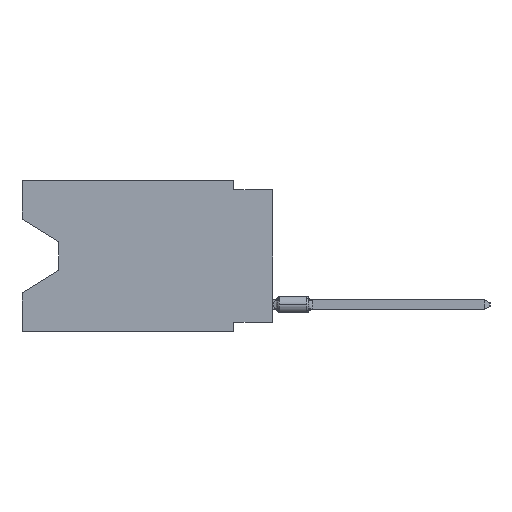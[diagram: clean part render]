
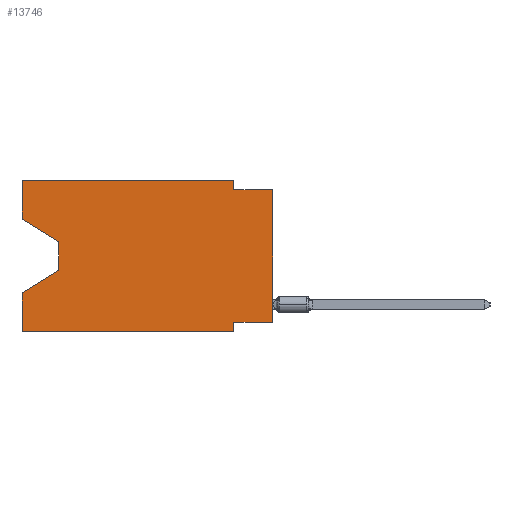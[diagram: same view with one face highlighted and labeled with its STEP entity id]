
A CAD part, left-side view. The second image highlights one B-rep face of the part: STEP entity #13746.
In plain terms, the highlighted planar face has unit normal (-1, 0, 0).
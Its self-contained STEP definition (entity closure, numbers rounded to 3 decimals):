
#204 = EDGE_CURVE ( 'NONE', #26065, #12717, #15722, .T. ) ;
#602 = VECTOR ( 'NONE', #33238, 1000. ) ;
#1590 = EDGE_CURVE ( 'NONE', #5926, #28278, #15044, .T. ) ;
#2101 = EDGE_CURVE ( 'NONE', #50760, #26065, #24980, .T. ) ;
#3023 = AXIS2_PLACEMENT_3D ( 'NONE', #23060, #48214, #26998 ) ;
#3065 = DIRECTION ( 'NONE',  ( 0., 1., 0. ) ) ;
#4132 = LINE ( 'NONE', #46897, #46453 ) ;
#4721 = ORIENTED_EDGE ( 'NONE', *, *, #204, .F. ) ;
#4770 = VECTOR ( 'NONE', #36698, 1000. ) ;
#5926 = VERTEX_POINT ( 'NONE', #23640 ) ;
#6097 = ORIENTED_EDGE ( 'NONE', *, *, #40734, .F. ) ;
#6844 = CARTESIAN_POINT ( 'NONE',  ( 0., 13.97, -5.893 ) ) ;
#7100 = ORIENTED_EDGE ( 'NONE', *, *, #37343, .T. ) ;
#8194 = DIRECTION ( 'NONE',  ( 0., -1., 0. ) ) ;
#9014 = DIRECTION ( 'NONE',  ( 0., 0., 1. ) ) ;
#9895 = EDGE_CURVE ( 'NONE', #27994, #50760, #37252, .T. ) ;
#10407 = CARTESIAN_POINT ( 'NONE',  ( 0., 0., -0.635 ) ) ;
#11821 = VECTOR ( 'NONE', #27916, 1000. ) ;
#12717 = VERTEX_POINT ( 'NONE', #54049 ) ;
#13085 = VERTEX_POINT ( 'NONE', #15163 ) ;
#13746 = ADVANCED_FACE ( 'NONE', ( #22240 ), #35372, .F. ) ;
#13950 = VECTOR ( 'NONE', #35538, 1000. ) ;
#14761 = CARTESIAN_POINT ( 'NONE',  ( 0., 0., -9.271 ) ) ;
#15003 = CARTESIAN_POINT ( 'NONE',  ( 0., 16.383, -9.906 ) ) ;
#15044 = LINE ( 'NONE', #49144, #11821 ) ;
#15163 = CARTESIAN_POINT ( 'NONE',  ( 0., 16.383, -2.546 ) ) ;
#15722 = LINE ( 'NONE', #10407, #52615 ) ;
#15752 = EDGE_CURVE ( 'NONE', #36811, #12717, #52286, .T. ) ;
#16286 = EDGE_CURVE ( 'NONE', #34697, #36162, #45864, .T. ) ;
#16830 = LINE ( 'NONE', #29154, #26396 ) ;
#16889 = VECTOR ( 'NONE', #38803, 1000. ) ;
#17072 = DIRECTION ( 'NONE',  ( 0., 0.855, -0.519 ) ) ;
#17743 = VECTOR ( 'NONE', #3065, 1000. ) ;
#20670 = DIRECTION ( 'NONE',  ( 0., 0., -1. ) ) ;
#21478 = LINE ( 'NONE', #42978, #16889 ) ;
#21681 = CARTESIAN_POINT ( 'NONE',  ( 0., 2.54, -9.906 ) ) ;
#21922 = ORIENTED_EDGE ( 'NONE', *, *, #9895, .F. ) ;
#22240 = FACE_OUTER_BOUND ( 'NONE', #24081, .T. ) ;
#22448 = VECTOR ( 'NONE', #28896, 1000. ) ;
#23060 = CARTESIAN_POINT ( 'NONE',  ( 0., 16.383, 0. ) ) ;
#23640 = CARTESIAN_POINT ( 'NONE',  ( 0., 2.54, -9.271 ) ) ;
#23828 = EDGE_CURVE ( 'NONE', #13085, #27994, #33508, .T. ) ;
#24081 = EDGE_LOOP ( 'NONE', ( #49636, #44207, #44071, #53375, #7100, #49864, #6097, #50116, #4721, #31886, #21922, #29466 ) ) ;
#24980 = LINE ( 'NONE', #37564, #22448 ) ;
#25000 = EDGE_CURVE ( 'NONE', #39496, #36162, #29987, .T. ) ;
#25499 = CARTESIAN_POINT ( 'NONE',  ( 0., 16.383, -7.36 ) ) ;
#26065 = VERTEX_POINT ( 'NONE', #30786 ) ;
#26396 = VECTOR ( 'NONE', #8194, 1000. ) ;
#26998 = DIRECTION ( 'NONE',  ( 0., 0., -1. ) ) ;
#27572 = CARTESIAN_POINT ( 'NONE',  ( 0., 16.383, 0. ) ) ;
#27916 = DIRECTION ( 'NONE',  ( 0., 0., -1. ) ) ;
#27994 = VERTEX_POINT ( 'NONE', #27572 ) ;
#28029 = CARTESIAN_POINT ( 'NONE',  ( 0., 16.383, 0. ) ) ;
#28278 = VERTEX_POINT ( 'NONE', #21681 ) ;
#28896 = DIRECTION ( 'NONE',  ( 0., 0., -1. ) ) ;
#29154 = CARTESIAN_POINT ( 'NONE',  ( 0., 16.383, -9.906 ) ) ;
#29466 = ORIENTED_EDGE ( 'NONE', *, *, #23828, .F. ) ;
#29987 = LINE ( 'NONE', #42824, #48081 ) ;
#30786 = CARTESIAN_POINT ( 'NONE',  ( 0., 2.54, -0.635 ) ) ;
#31886 = ORIENTED_EDGE ( 'NONE', *, *, #2101, .F. ) ;
#32771 = DIRECTION ( 'NONE',  ( 0., -1., 0. ) ) ;
#33238 = DIRECTION ( 'NONE',  ( 0., 0., 1. ) ) ;
#33508 = LINE ( 'NONE', #54151, #602 ) ;
#34697 = VERTEX_POINT ( 'NONE', #6844 ) ;
#35372 = PLANE ( 'NONE',  #3023 ) ;
#35538 = DIRECTION ( 'NONE',  ( 0., 0., 1. ) ) ;
#36162 = VERTEX_POINT ( 'NONE', #25499 ) ;
#36698 = DIRECTION ( 'NONE',  ( 0., -1., 0. ) ) ;
#36811 = VERTEX_POINT ( 'NONE', #14761 ) ;
#37252 = LINE ( 'NONE', #28029, #4770 ) ;
#37343 = EDGE_CURVE ( 'NONE', #39496, #28278, #16830, .T. ) ;
#37564 = CARTESIAN_POINT ( 'NONE',  ( 0., 2.54, 0. ) ) ;
#38803 = DIRECTION ( 'NONE',  ( 0., -0.855, -0.519 ) ) ;
#39278 = VERTEX_POINT ( 'NONE', #49313 ) ;
#39496 = VERTEX_POINT ( 'NONE', #15003 ) ;
#40552 = VECTOR ( 'NONE', #17072, 1000. ) ;
#40734 = EDGE_CURVE ( 'NONE', #36811, #5926, #50017, .T. ) ;
#41649 = CARTESIAN_POINT ( 'NONE',  ( 0., 0., -9.271 ) ) ;
#42494 = CARTESIAN_POINT ( 'NONE',  ( 0., 13.97, -5.893 ) ) ;
#42824 = CARTESIAN_POINT ( 'NONE',  ( 0., 16.383, 0. ) ) ;
#42978 = CARTESIAN_POINT ( 'NONE',  ( 0., 16.383, -2.546 ) ) ;
#43487 = CARTESIAN_POINT ( 'NONE',  ( 0., 2.54, 0. ) ) ;
#44071 = ORIENTED_EDGE ( 'NONE', *, *, #16286, .T. ) ;
#44207 = ORIENTED_EDGE ( 'NONE', *, *, #48361, .T. ) ;
#45864 = LINE ( 'NONE', #42494, #40552 ) ;
#46453 = VECTOR ( 'NONE', #20670, 1000. ) ;
#46897 = CARTESIAN_POINT ( 'NONE',  ( 0., 13.97, -4.013 ) ) ;
#48081 = VECTOR ( 'NONE', #9014, 1000. ) ;
#48214 = DIRECTION ( 'NONE',  ( 1., 0., 0. ) ) ;
#48361 = EDGE_CURVE ( 'NONE', #39278, #34697, #4132, .T. ) ;
#49144 = CARTESIAN_POINT ( 'NONE',  ( 0., 2.54, -9.906 ) ) ;
#49313 = CARTESIAN_POINT ( 'NONE',  ( 0., 13.97, -4.013 ) ) ;
#49636 = ORIENTED_EDGE ( 'NONE', *, *, #52405, .T. ) ;
#49864 = ORIENTED_EDGE ( 'NONE', *, *, #1590, .F. ) ;
#50017 = LINE ( 'NONE', #41649, #17743 ) ;
#50116 = ORIENTED_EDGE ( 'NONE', *, *, #15752, .T. ) ;
#50760 = VERTEX_POINT ( 'NONE', #43487 ) ;
#52286 = LINE ( 'NONE', #53124, #13950 ) ;
#52405 = EDGE_CURVE ( 'NONE', #13085, #39278, #21478, .T. ) ;
#52615 = VECTOR ( 'NONE', #32771, 1000. ) ;
#53124 = CARTESIAN_POINT ( 'NONE',  ( 0., 0., 0. ) ) ;
#53375 = ORIENTED_EDGE ( 'NONE', *, *, #25000, .F. ) ;
#54049 = CARTESIAN_POINT ( 'NONE',  ( 0., 0., -0.635 ) ) ;
#54151 = CARTESIAN_POINT ( 'NONE',  ( 0., 16.383, 0. ) ) ;
